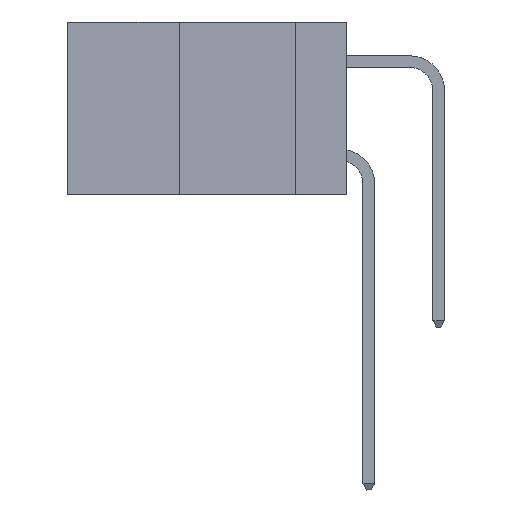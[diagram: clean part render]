
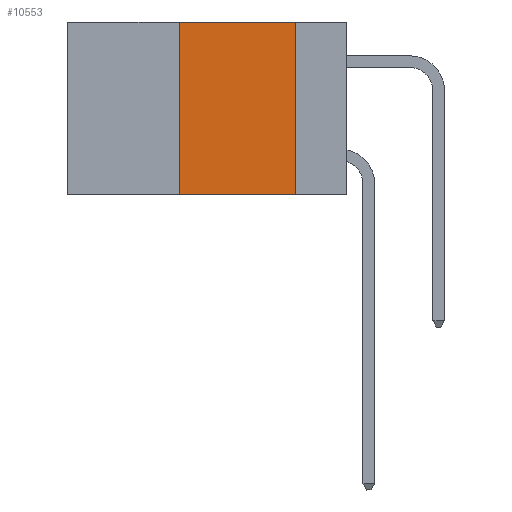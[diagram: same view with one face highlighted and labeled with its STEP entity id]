
A CAD part, left-side view. The second image highlights one B-rep face of the part: STEP entity #10553.
In plain terms, the highlighted planar face has unit normal (-1, 0, 0).
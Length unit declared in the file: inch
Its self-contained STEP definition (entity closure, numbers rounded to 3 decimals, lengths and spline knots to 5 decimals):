
#941 = ORIENTED_EDGE ( 'NONE', *, *, #26335, .F. ) ;
#1500 = CARTESIAN_POINT ( 'NONE',  ( 0., 0.11, -0.37 ) ) ;
#3012 = VECTOR ( 'NONE', #28764, 39.37008 ) ;
#4868 = CARTESIAN_POINT ( 'NONE',  ( 0., 0.11, 0. ) ) ;
#5621 = CARTESIAN_POINT ( 'NONE',  ( 0., 0.36, 0. ) ) ;
#6075 = PLANE ( 'NONE',  #17480 ) ;
#8053 = VERTEX_POINT ( 'NONE', #4868 ) ;
#10553 = ADVANCED_FACE ( 'NONE', ( #32463 ), #6075, .F. ) ;
#10796 = CARTESIAN_POINT ( 'NONE',  ( 0., 0.6, -0.37 ) ) ;
#11059 = EDGE_CURVE ( 'NONE', #32802, #29602, #24917, .T. ) ;
#12981 = LINE ( 'NONE', #34676, #35765 ) ;
#14814 = CARTESIAN_POINT ( 'NONE',  ( 0., 0.6, 0. ) ) ;
#14884 = EDGE_CURVE ( 'NONE', #32802, #19959, #29605, .T. ) ;
#16542 = ORIENTED_EDGE ( 'NONE', *, *, #11059, .T. ) ;
#17480 = AXIS2_PLACEMENT_3D ( 'NONE', #27010, #36133, #24140 ) ;
#18729 = ORIENTED_EDGE ( 'NONE', *, *, #32598, .F. ) ;
#19959 = VERTEX_POINT ( 'NONE', #36748 ) ;
#21211 = DIRECTION ( 'NONE',  ( 0., 0., 1. ) ) ;
#23361 = LINE ( 'NONE', #14814, #27046 ) ;
#24140 = DIRECTION ( 'NONE',  ( 0., 0., -1. ) ) ;
#24917 = LINE ( 'NONE', #10796, #3012 ) ;
#26335 = EDGE_CURVE ( 'NONE', #19959, #8053, #23361, .T. ) ;
#27010 = CARTESIAN_POINT ( 'NONE',  ( 0., 0.6, 0. ) ) ;
#27046 = VECTOR ( 'NONE', #35618, 39.37008 ) ;
#28764 = DIRECTION ( 'NONE',  ( 0., -1., 0. ) ) ;
#29602 = VERTEX_POINT ( 'NONE', #1500 ) ;
#29605 = LINE ( 'NONE', #5621, #31520 ) ;
#31520 = VECTOR ( 'NONE', #21211, 39.37008 ) ;
#31917 = DIRECTION ( 'NONE',  ( 0., 0., -1. ) ) ;
#32463 = FACE_OUTER_BOUND ( 'NONE', #37806, .T. ) ;
#32598 = EDGE_CURVE ( 'NONE', #8053, #29602, #12981, .T. ) ;
#32802 = VERTEX_POINT ( 'NONE', #38290 ) ;
#34676 = CARTESIAN_POINT ( 'NONE',  ( 0., 0.11, 0. ) ) ;
#35579 = ORIENTED_EDGE ( 'NONE', *, *, #14884, .F. ) ;
#35618 = DIRECTION ( 'NONE',  ( 0., -1., 0. ) ) ;
#35765 = VECTOR ( 'NONE', #31917, 39.37008 ) ;
#36133 = DIRECTION ( 'NONE',  ( 1., 0., 0. ) ) ;
#36748 = CARTESIAN_POINT ( 'NONE',  ( 0., 0.36, 0. ) ) ;
#37806 = EDGE_LOOP ( 'NONE', ( #18729, #941, #35579, #16542 ) ) ;
#38290 = CARTESIAN_POINT ( 'NONE',  ( 0., 0.36, -0.37 ) ) ;
